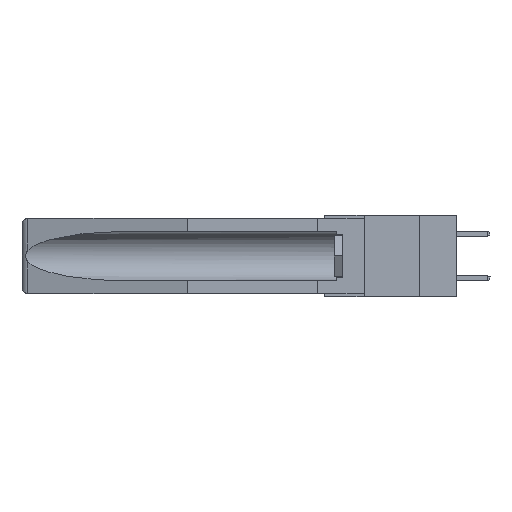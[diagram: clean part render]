
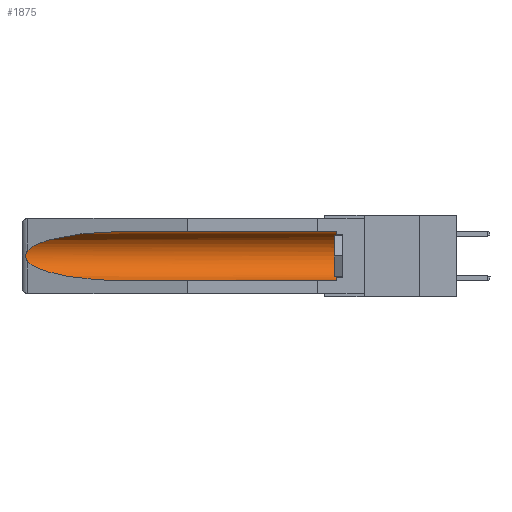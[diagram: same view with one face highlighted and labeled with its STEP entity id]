
A CAD part, left-side view. The second image highlights one B-rep face of the part: STEP entity #1875.
In plain terms, the highlighted cylindrical face has radius 2.857 mm (diameter 5.715 mm), a partial arc.
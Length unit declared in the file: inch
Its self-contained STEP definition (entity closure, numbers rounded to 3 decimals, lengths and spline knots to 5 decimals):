
#103 = EDGE_LOOP ( 'NONE', ( #14557, #9226, #9739, #1759, #16793, #8196 ) ) ;
#924 = AXIS2_PLACEMENT_3D ( 'NONE', #9583, #15035, #6992 ) ;
#1367 = DIRECTION ( 'NONE',  ( 0., 1., 0. ) ) ;
#1394 = CYLINDRICAL_SURFACE ( 'NONE', #15638, 0.1125 ) ;
#1581 = EDGE_CURVE ( 'NONE', #15450, #16389, #14104, .T. ) ;
#1719 = EDGE_CURVE ( 'NONE', #9487, #5218, #7967, .T. ) ;
#1759 = ORIENTED_EDGE ( 'NONE', *, *, #15510, .F. ) ;
#1875 = ADVANCED_FACE ( 'NONE', ( #4177 ), #1394, .F. ) ;
#2192 = VECTOR ( 'NONE', #6348, 39.37008 ) ;
#2879 = VECTOR ( 'NONE', #1367, 39.37008 ) ;
#3235 = CARTESIAN_POINT ( 'NONE',  ( 0.155, -0.30754, -0.1715 ) ) ;
#4177 = FACE_OUTER_BOUND ( 'NONE', #103, .T. ) ;
#4206 =( BOUNDED_CURVE ( )  B_SPLINE_CURVE ( 3, ( #11987, #13013, #16148, #13416 ),
 .UNSPECIFIED., .F., .F. ) 
 B_SPLINE_CURVE_WITH_KNOTS ( ( 4, 4 ),
 ( 4.71239, 6.08839 ),
 .UNSPECIFIED. ) 
 CURVE ( )  GEOMETRIC_REPRESENTATION_ITEM ( )  RATIONAL_B_SPLINE_CURVE ( ( 1., 0.848, 0.848, 1. ) ) 
 REPRESENTATION_ITEM ( '' )  );
#4260 = CARTESIAN_POINT ( 'NONE',  ( 0.26537, 1.52718, -0.14972 ) ) ;
#4811 = CARTESIAN_POINT ( 'NONE',  ( 0.26537, 1.52718, -0.19328 ) ) ;
#5218 = VERTEX_POINT ( 'NONE', #15691 ) ;
#5651 = CARTESIAN_POINT ( 'NONE',  ( 0.26597, 1.52961, -0.15275 ) ) ;
#5823 = CARTESIAN_POINT ( 'NONE',  ( 0.2673, 1.53269, -0.17917 ) ) ;
#6304 =( BOUNDED_CURVE ( )  B_SPLINE_CURVE ( 3, ( #4811, #17148, #17323, #14499 ),
 .UNSPECIFIED., .F., .F. ) 
 B_SPLINE_CURVE_WITH_KNOTS ( ( 4, 4 ),
 ( 0.1948, 1.5708 ),
 .UNSPECIFIED. ) 
 CURVE ( )  GEOMETRIC_REPRESENTATION_ITEM ( )  RATIONAL_B_SPLINE_CURVE ( ( 1., 0.848, 0.848, 1. ) ) 
 REPRESENTATION_ITEM ( '' )  );
#6348 = DIRECTION ( 'NONE',  ( 0., 1., 0. ) ) ;
#6838 = CARTESIAN_POINT ( 'NONE',  ( 0.155, -0.30754, -0.059 ) ) ;
#6992 = DIRECTION ( 'NONE',  ( 0., 0., 1. ) ) ;
#7042 = CARTESIAN_POINT ( 'NONE',  ( 0.2673, 1.5327, -0.16383 ) ) ;
#7967 = B_SPLINE_CURVE_WITH_KNOTS ( 'NONE', 3,
 ( #4260, #5651, #14095, #7042, #11209, #12589, #5823, #15452, #13981, #16694 ),
 .UNSPECIFIED., .F., .F.,
 ( 4, 2, 2, 2, 4 ),
 ( 0., 0.00029, 0.00058, 0.00087, 0.00117 ),
 .UNSPECIFIED. ) ;
#8196 = ORIENTED_EDGE ( 'NONE', *, *, #1581, .T. ) ;
#8744 = DIRECTION ( 'NONE',  ( 0., 1., 0. ) ) ;
#9226 = ORIENTED_EDGE ( 'NONE', *, *, #1719, .T. ) ;
#9487 = VERTEX_POINT ( 'NONE', #16583 ) ;
#9583 = CARTESIAN_POINT ( 'NONE',  ( 0.155, 0.126, -0.1715 ) ) ;
#9739 = ORIENTED_EDGE ( 'NONE', *, *, #13174, .T. ) ;
#10537 = CIRCLE ( 'NONE', #924, 0.1125 ) ;
#11209 = CARTESIAN_POINT ( 'NONE',  ( 0.2675, 1.53308, -0.16763 ) ) ;
#11572 = DIRECTION ( 'NONE',  ( 0., 0., 1. ) ) ;
#11987 = CARTESIAN_POINT ( 'NONE',  ( 0.155, 1.07973, -0.059 ) ) ;
#12121 = CARTESIAN_POINT ( 'NONE',  ( 0.155, -0.30754, -0.284 ) ) ;
#12589 = CARTESIAN_POINT ( 'NONE',  ( 0.2675, 1.53308, -0.17534 ) ) ;
#13013 = CARTESIAN_POINT ( 'NONE',  ( 0.21114, 1.30732, -0.059 ) ) ;
#13174 = EDGE_CURVE ( 'NONE', #5218, #15558, #6304, .T. ) ;
#13416 = CARTESIAN_POINT ( 'NONE',  ( 0.26537, 1.52718, -0.14972 ) ) ;
#13515 = EDGE_CURVE ( 'NONE', #14461, #15450, #10537, .T. ) ;
#13954 = CARTESIAN_POINT ( 'NONE',  ( 0.155, 1.07973, -0.059 ) ) ;
#13981 = CARTESIAN_POINT ( 'NONE',  ( 0.26597, 1.5296, -0.19026 ) ) ;
#14095 = CARTESIAN_POINT ( 'NONE',  ( 0.26654, 1.53092, -0.15636 ) ) ;
#14104 = LINE ( 'NONE', #6838, #2879 ) ;
#14461 = VERTEX_POINT ( 'NONE', #16326 ) ;
#14499 = CARTESIAN_POINT ( 'NONE',  ( 0.155, 1.07973, -0.284 ) ) ;
#14557 = ORIENTED_EDGE ( 'NONE', *, *, #17200, .T. ) ;
#14799 = CARTESIAN_POINT ( 'NONE',  ( 0.155, 1.07973, -0.284 ) ) ;
#15035 = DIRECTION ( 'NONE',  ( 0., -1., 0. ) ) ;
#15450 = VERTEX_POINT ( 'NONE', #17648 ) ;
#15452 = CARTESIAN_POINT ( 'NONE',  ( 0.26655, 1.53094, -0.18657 ) ) ;
#15510 = EDGE_CURVE ( 'NONE', #14461, #15558, #15545, .T. ) ;
#15545 = LINE ( 'NONE', #12121, #2192 ) ;
#15558 = VERTEX_POINT ( 'NONE', #14799 ) ;
#15638 = AXIS2_PLACEMENT_3D ( 'NONE', #3235, #8744, #11572 ) ;
#15691 = CARTESIAN_POINT ( 'NONE',  ( 0.26537, 1.52718, -0.19328 ) ) ;
#16148 = CARTESIAN_POINT ( 'NONE',  ( 0.25451, 1.48313, -0.09465 ) ) ;
#16326 = CARTESIAN_POINT ( 'NONE',  ( 0.155, 0.126, -0.284 ) ) ;
#16389 = VERTEX_POINT ( 'NONE', #13954 ) ;
#16583 = CARTESIAN_POINT ( 'NONE',  ( 0.26537, 1.52718, -0.14972 ) ) ;
#16694 = CARTESIAN_POINT ( 'NONE',  ( 0.26537, 1.52718, -0.19328 ) ) ;
#16793 = ORIENTED_EDGE ( 'NONE', *, *, #13515, .T. ) ;
#17148 = CARTESIAN_POINT ( 'NONE',  ( 0.25451, 1.48313, -0.24835 ) ) ;
#17200 = EDGE_CURVE ( 'NONE', #16389, #9487, #4206, .T. ) ;
#17323 = CARTESIAN_POINT ( 'NONE',  ( 0.21114, 1.30732, -0.284 ) ) ;
#17648 = CARTESIAN_POINT ( 'NONE',  ( 0.155, 0.126, -0.059 ) ) ;
